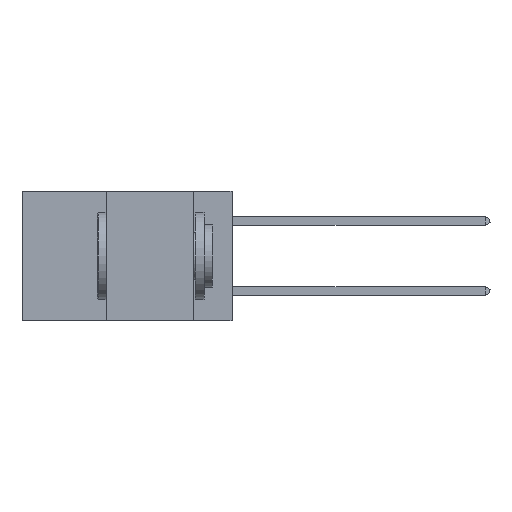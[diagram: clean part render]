
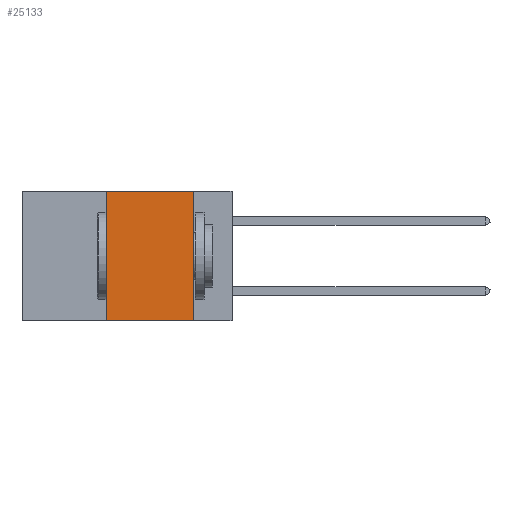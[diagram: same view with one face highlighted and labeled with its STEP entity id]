
A CAD part, left-side view. The second image highlights one B-rep face of the part: STEP entity #25133.
In plain terms, the highlighted planar face has unit normal (-1, 0, 0).
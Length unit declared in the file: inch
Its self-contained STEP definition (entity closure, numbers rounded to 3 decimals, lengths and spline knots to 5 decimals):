
#114 = EDGE_CURVE ( 'NONE', #2041, #35882, #34599, .T. ) ;
#1754 = DIRECTION ( 'NONE',  ( 1., 0., 0. ) ) ;
#1790 = VERTEX_POINT ( 'NONE', #10805 ) ;
#2041 = VERTEX_POINT ( 'NONE', #43027 ) ;
#5068 = PLANE ( 'NONE',  #21185 ) ;
#5918 = EDGE_LOOP ( 'NONE', ( #10093, #12268, #30674, #6343 ) ) ;
#6343 = ORIENTED_EDGE ( 'NONE', *, *, #31073, .T. ) ;
#6907 = DIRECTION ( 'NONE',  ( 0., -1., 0. ) ) ;
#8320 = VECTOR ( 'NONE', #35715, 39.37008 ) ;
#10093 = ORIENTED_EDGE ( 'NONE', *, *, #16307, .F. ) ;
#10557 = FACE_OUTER_BOUND ( 'NONE', #5918, .T. ) ;
#10805 = CARTESIAN_POINT ( 'NONE',  ( 0., 0.11, -0.37 ) ) ;
#10876 = LINE ( 'NONE', #41267, #18966 ) ;
#12268 = ORIENTED_EDGE ( 'NONE', *, *, #28828, .F. ) ;
#15702 = VERTEX_POINT ( 'NONE', #22333 ) ;
#16307 = EDGE_CURVE ( 'NONE', #15702, #1790, #17492, .T. ) ;
#17492 = LINE ( 'NONE', #21834, #8320 ) ;
#18966 = VECTOR ( 'NONE', #6907, 39.37008 ) ;
#19453 = VECTOR ( 'NONE', #41470, 39.37008 ) ;
#21185 = AXIS2_PLACEMENT_3D ( 'NONE', #43030, #1754, #25901 ) ;
#21834 = CARTESIAN_POINT ( 'NONE',  ( 0., 0.11, 0. ) ) ;
#22333 = CARTESIAN_POINT ( 'NONE',  ( 0., 0.11, 0. ) ) ;
#25133 = ADVANCED_FACE ( 'NONE', ( #10557 ), #5068, .F. ) ;
#25421 = VECTOR ( 'NONE', #32826, 39.37008 ) ;
#25901 = DIRECTION ( 'NONE',  ( 0., 0., -1. ) ) ;
#27642 = CARTESIAN_POINT ( 'NONE',  ( 0., 0.6, 0. ) ) ;
#28070 = CARTESIAN_POINT ( 'NONE',  ( 0., 0.36, 0. ) ) ;
#28673 = LINE ( 'NONE', #27642, #19453 ) ;
#28828 = EDGE_CURVE ( 'NONE', #35882, #15702, #28673, .T. ) ;
#30674 = ORIENTED_EDGE ( 'NONE', *, *, #114, .F. ) ;
#31073 = EDGE_CURVE ( 'NONE', #2041, #1790, #10876, .T. ) ;
#32826 = DIRECTION ( 'NONE',  ( 0., 0., 1. ) ) ;
#34599 = LINE ( 'NONE', #42874, #25421 ) ;
#35715 = DIRECTION ( 'NONE',  ( 0., 0., -1. ) ) ;
#35882 = VERTEX_POINT ( 'NONE', #28070 ) ;
#41267 = CARTESIAN_POINT ( 'NONE',  ( 0., 0.6, -0.37 ) ) ;
#41470 = DIRECTION ( 'NONE',  ( 0., -1., 0. ) ) ;
#42874 = CARTESIAN_POINT ( 'NONE',  ( 0., 0.36, 0. ) ) ;
#43027 = CARTESIAN_POINT ( 'NONE',  ( 0., 0.36, -0.37 ) ) ;
#43030 = CARTESIAN_POINT ( 'NONE',  ( 0., 0.6, 0. ) ) ;
